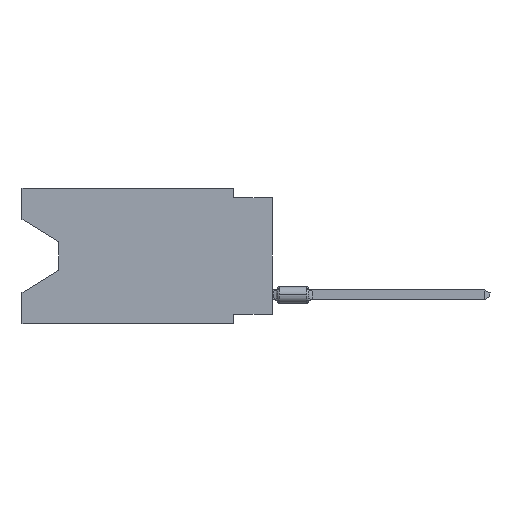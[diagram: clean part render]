
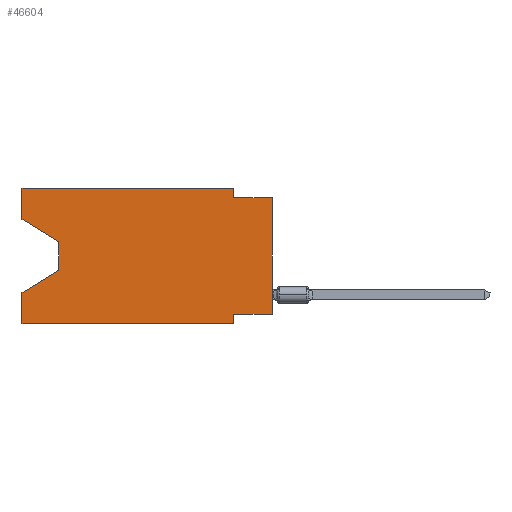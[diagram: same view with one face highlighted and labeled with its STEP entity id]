
A CAD part, left-side view. The second image highlights one B-rep face of the part: STEP entity #46604.
In plain terms, the highlighted planar face has unit normal (-1, 0, 0).
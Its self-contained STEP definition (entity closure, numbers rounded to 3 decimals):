
#7 = LINE ( 'NONE', #36474, #3883 ) ;
#449 = LINE ( 'NONE', #93241, #61996 ) ;
#775 = ORIENTED_EDGE ( 'NONE', *, *, #9529, .T. ) ;
#1729 = CARTESIAN_POINT ( 'NONE',  ( 0., 13.97, -3.505 ) ) ;
#2699 = CARTESIAN_POINT ( 'NONE',  ( 0., 13.97, -5.385 ) ) ;
#2815 = CARTESIAN_POINT ( 'NONE',  ( 0., 2.54, -8.89 ) ) ;
#3020 = CARTESIAN_POINT ( 'NONE',  ( 0., 2.54, -8.255 ) ) ;
#3029 = DIRECTION ( 'NONE',  ( 0., -1., 0. ) ) ;
#3042 = FACE_OUTER_BOUND ( 'NONE', #68576, .T. ) ;
#3883 = VECTOR ( 'NONE', #85240, 1000. ) ;
#4484 = CARTESIAN_POINT ( 'NONE',  ( 0., 0., -8.255 ) ) ;
#5567 = ORIENTED_EDGE ( 'NONE', *, *, #26296, .T. ) ;
#6969 = EDGE_CURVE ( 'NONE', #56119, #42726, #22743, .T. ) ;
#6974 = CARTESIAN_POINT ( 'NONE',  ( 0., 16.383, -6.852 ) ) ;
#8330 = VECTOR ( 'NONE', #44689, 1000. ) ;
#9529 = EDGE_CURVE ( 'NONE', #23717, #64955, #58111, .T. ) ;
#13531 = VERTEX_POINT ( 'NONE', #3020 ) ;
#13774 = CARTESIAN_POINT ( 'NONE',  ( 0., 16.383, 0. ) ) ;
#14446 = DIRECTION ( 'NONE',  ( 0., -0.855, -0.519 ) ) ;
#15705 = VECTOR ( 'NONE', #80958, 1000. ) ;
#16444 = EDGE_CURVE ( 'NONE', #41788, #33067, #82514, .T. ) ;
#16559 = CARTESIAN_POINT ( 'NONE',  ( 0., 2.54, 0. ) ) ;
#18176 = AXIS2_PLACEMENT_3D ( 'NONE', #31969, #89665, #53733 ) ;
#19020 = CARTESIAN_POINT ( 'NONE',  ( 0., 0., -0.635 ) ) ;
#22743 = LINE ( 'NONE', #13774, #15705 ) ;
#23369 = CARTESIAN_POINT ( 'NONE',  ( 0., 16.383, -8.89 ) ) ;
#23553 = DIRECTION ( 'NONE',  ( 0., 0., 1. ) ) ;
#23717 = VERTEX_POINT ( 'NONE', #48177 ) ;
#23843 = DIRECTION ( 'NONE',  ( 0., -1., 0. ) ) ;
#23935 = ORIENTED_EDGE ( 'NONE', *, *, #45606, .T. ) ;
#26296 = EDGE_CURVE ( 'NONE', #34532, #33067, #7, .T. ) ;
#28161 = LINE ( 'NONE', #23369, #48363 ) ;
#29142 = CARTESIAN_POINT ( 'NONE',  ( 0., 16.383, -2.038 ) ) ;
#29942 = CARTESIAN_POINT ( 'NONE',  ( 0., 16.383, 0. ) ) ;
#30076 = LINE ( 'NONE', #29142, #86259 ) ;
#31010 = CARTESIAN_POINT ( 'NONE',  ( 0., 0., -0.635 ) ) ;
#31639 = CARTESIAN_POINT ( 'NONE',  ( 0., 16.383, -2.038 ) ) ;
#31969 = CARTESIAN_POINT ( 'NONE',  ( 0., 16.383, 0. ) ) ;
#32485 = DIRECTION ( 'NONE',  ( 0., 1., 0. ) ) ;
#32834 = CARTESIAN_POINT ( 'NONE',  ( 0., 16.383, 0. ) ) ;
#33067 = VERTEX_POINT ( 'NONE', #6974 ) ;
#34063 = EDGE_CURVE ( 'NONE', #13531, #41644, #38827, .T. ) ;
#34457 = ORIENTED_EDGE ( 'NONE', *, *, #48515, .F. ) ;
#34532 = VERTEX_POINT ( 'NONE', #2699 ) ;
#34566 = ORIENTED_EDGE ( 'NONE', *, *, #16444, .F. ) ;
#36188 = ORIENTED_EDGE ( 'NONE', *, *, #68736, .F. ) ;
#36474 = CARTESIAN_POINT ( 'NONE',  ( 0., 13.97, -5.385 ) ) ;
#37381 = DIRECTION ( 'NONE',  ( 0., 0., 1. ) ) ;
#37762 = CARTESIAN_POINT ( 'NONE',  ( 0., 0., 0. ) ) ;
#38827 = LINE ( 'NONE', #2815, #45784 ) ;
#39578 = LINE ( 'NONE', #4484, #44596 ) ;
#41644 = VERTEX_POINT ( 'NONE', #74161 ) ;
#41788 = VERTEX_POINT ( 'NONE', #49996 ) ;
#42726 = VERTEX_POINT ( 'NONE', #16559 ) ;
#42854 = VERTEX_POINT ( 'NONE', #53509 ) ;
#44106 = ORIENTED_EDGE ( 'NONE', *, *, #55269, .F. ) ;
#44596 = VECTOR ( 'NONE', #32485, 1000. ) ;
#44689 = DIRECTION ( 'NONE',  ( 0., 0., -1. ) ) ;
#44940 = VECTOR ( 'NONE', #23553, 1000. ) ;
#45606 = EDGE_CURVE ( 'NONE', #89612, #93168, #30076, .T. ) ;
#45697 = PLANE ( 'NONE',  #18176 ) ;
#45784 = VECTOR ( 'NONE', #52552, 1000. ) ;
#46604 = ADVANCED_FACE ( 'NONE', ( #3042 ), #45697, .F. ) ;
#46734 = CARTESIAN_POINT ( 'NONE',  ( 0., 13.97, -3.505 ) ) ;
#47050 = VECTOR ( 'NONE', #91458, 1000. ) ;
#47652 = LINE ( 'NONE', #46734, #61865 ) ;
#48177 = CARTESIAN_POINT ( 'NONE',  ( 0., 0., -8.255 ) ) ;
#48348 = EDGE_CURVE ( 'NONE', #23717, #13531, #39578, .T. ) ;
#48363 = VECTOR ( 'NONE', #23843, 1000. ) ;
#48515 = EDGE_CURVE ( 'NONE', #42726, #42854, #80161, .T. ) ;
#49996 = CARTESIAN_POINT ( 'NONE',  ( 0., 16.383, -8.89 ) ) ;
#52552 = DIRECTION ( 'NONE',  ( 0., 0., -1. ) ) ;
#52739 = EDGE_CURVE ( 'NONE', #93168, #34532, #47652, .T. ) ;
#53509 = CARTESIAN_POINT ( 'NONE',  ( 0., 2.54, -0.635 ) ) ;
#53733 = DIRECTION ( 'NONE',  ( 0., 0., -1. ) ) ;
#55269 = EDGE_CURVE ( 'NONE', #89612, #56119, #449, .T. ) ;
#56119 = VERTEX_POINT ( 'NONE', #29942 ) ;
#58111 = LINE ( 'NONE', #37762, #44940 ) ;
#59341 = CARTESIAN_POINT ( 'NONE',  ( 0., 2.54, 0. ) ) ;
#61865 = VECTOR ( 'NONE', #67531, 1000. ) ;
#61996 = VECTOR ( 'NONE', #37381, 1000. ) ;
#64228 = ORIENTED_EDGE ( 'NONE', *, *, #34063, .F. ) ;
#64955 = VERTEX_POINT ( 'NONE', #19020 ) ;
#66566 = ORIENTED_EDGE ( 'NONE', *, *, #80392, .T. ) ;
#67531 = DIRECTION ( 'NONE',  ( 0., 0., -1. ) ) ;
#68535 = ORIENTED_EDGE ( 'NONE', *, *, #52739, .T. ) ;
#68576 = EDGE_LOOP ( 'NONE', ( #23935, #68535, #5567, #34566, #66566, #64228, #85876, #775, #36188, #34457, #88782, #44106 ) ) ;
#68736 = EDGE_CURVE ( 'NONE', #42854, #64955, #88237, .T. ) ;
#72953 = VECTOR ( 'NONE', #3029, 1000. ) ;
#74161 = CARTESIAN_POINT ( 'NONE',  ( 0., 2.54, -8.89 ) ) ;
#80161 = LINE ( 'NONE', #59341, #8330 ) ;
#80392 = EDGE_CURVE ( 'NONE', #41788, #41644, #28161, .T. ) ;
#80958 = DIRECTION ( 'NONE',  ( 0., -1., 0. ) ) ;
#82514 = LINE ( 'NONE', #32834, #47050 ) ;
#85240 = DIRECTION ( 'NONE',  ( 0., 0.855, -0.519 ) ) ;
#85876 = ORIENTED_EDGE ( 'NONE', *, *, #48348, .F. ) ;
#86259 = VECTOR ( 'NONE', #14446, 1000. ) ;
#88237 = LINE ( 'NONE', #31010, #72953 ) ;
#88782 = ORIENTED_EDGE ( 'NONE', *, *, #6969, .F. ) ;
#89612 = VERTEX_POINT ( 'NONE', #31639 ) ;
#89665 = DIRECTION ( 'NONE',  ( 1., 0., 0. ) ) ;
#91458 = DIRECTION ( 'NONE',  ( 0., 0., 1. ) ) ;
#93168 = VERTEX_POINT ( 'NONE', #1729 ) ;
#93241 = CARTESIAN_POINT ( 'NONE',  ( 0., 16.383, 0. ) ) ;
